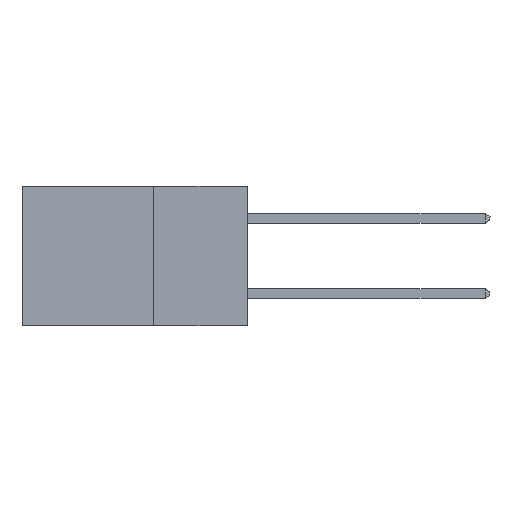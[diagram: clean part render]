
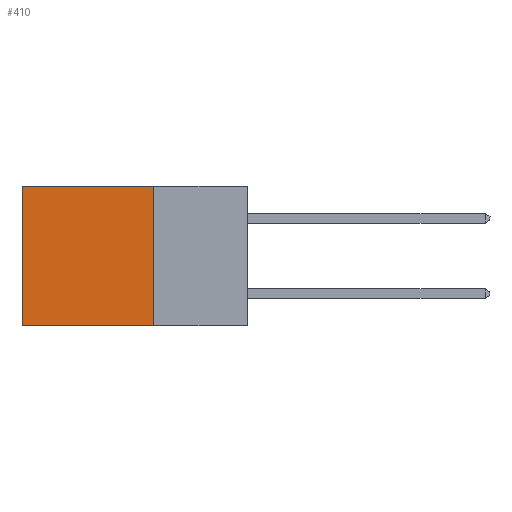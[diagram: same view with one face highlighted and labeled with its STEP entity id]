
A CAD part, left-side view. The second image highlights one B-rep face of the part: STEP entity #410.
In plain terms, the highlighted planar face has unit normal (-1, 0, 0).
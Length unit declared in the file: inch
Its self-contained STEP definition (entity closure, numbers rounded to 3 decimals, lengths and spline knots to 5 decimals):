
#233 = EDGE_CURVE ( 'NONE', #3454, #2175, #1921, .T. ) ;
#367 = DIRECTION ( 'NONE',  ( 0., 0., -1. ) ) ;
#410 = ADVANCED_FACE ( 'NONE', ( #2088 ), #538, .F. ) ;
#538 = PLANE ( 'NONE',  #8859 ) ;
#594 = VECTOR ( 'NONE', #7044, 39.37008 ) ;
#1869 = CARTESIAN_POINT ( 'NONE',  ( 0.2615, 0.6, 0. ) ) ;
#1921 = LINE ( 'NONE', #4471, #6898 ) ;
#2067 = LINE ( 'NONE', #2833, #594 ) ;
#2088 = FACE_OUTER_BOUND ( 'NONE', #9900, .T. ) ;
#2175 = VERTEX_POINT ( 'NONE', #5304 ) ;
#2203 = DIRECTION ( 'NONE',  ( 1., 0., 0. ) ) ;
#2833 = CARTESIAN_POINT ( 'NONE',  ( 0.2615, 0.6, -0.37 ) ) ;
#3124 = VECTOR ( 'NONE', #7638, 39.37008 ) ;
#3249 = EDGE_CURVE ( 'NONE', #3454, #9092, #9214, .T. ) ;
#3454 = VERTEX_POINT ( 'NONE', #5365 ) ;
#4315 = CARTESIAN_POINT ( 'NONE',  ( 0.2615, 0.25, -0.37 ) ) ;
#4471 = CARTESIAN_POINT ( 'NONE',  ( 0.2615, 0.25, -0.37 ) ) ;
#4702 = ORIENTED_EDGE ( 'NONE', *, *, #5104, .F. ) ;
#4731 = CARTESIAN_POINT ( 'NONE',  ( 0.2615, 0.6, -0.37 ) ) ;
#5104 = EDGE_CURVE ( 'NONE', #2175, #7951, #9910, .T. ) ;
#5304 = CARTESIAN_POINT ( 'NONE',  ( 0.2615, 0.25, -0.37 ) ) ;
#5365 = CARTESIAN_POINT ( 'NONE',  ( 0.2615, 0.25, 0. ) ) ;
#5917 = DIRECTION ( 'NONE',  ( 0., 1., 0. ) ) ;
#6229 = ORIENTED_EDGE ( 'NONE', *, *, #3249, .T. ) ;
#6306 = ORIENTED_EDGE ( 'NONE', *, *, #233, .F. ) ;
#6898 = VECTOR ( 'NONE', #6980, 39.37008 ) ;
#6980 = DIRECTION ( 'NONE',  ( 0., 0., -1. ) ) ;
#7044 = DIRECTION ( 'NONE',  ( 0., 0., -1. ) ) ;
#7065 = VECTOR ( 'NONE', #5917, 39.37008 ) ;
#7638 = DIRECTION ( 'NONE',  ( 0., 1., 0. ) ) ;
#7951 = VERTEX_POINT ( 'NONE', #4731 ) ;
#8197 = EDGE_CURVE ( 'NONE', #9092, #7951, #2067, .T. ) ;
#8536 = ORIENTED_EDGE ( 'NONE', *, *, #8197, .T. ) ;
#8859 = AXIS2_PLACEMENT_3D ( 'NONE', #10464, #2203, #367 ) ;
#9057 = CARTESIAN_POINT ( 'NONE',  ( 0.2615, 0.25, 0. ) ) ;
#9092 = VERTEX_POINT ( 'NONE', #1869 ) ;
#9214 = LINE ( 'NONE', #9057, #7065 ) ;
#9900 = EDGE_LOOP ( 'NONE', ( #8536, #4702, #6306, #6229 ) ) ;
#9910 = LINE ( 'NONE', #4315, #3124 ) ;
#10464 = CARTESIAN_POINT ( 'NONE',  ( 0.2615, 0.25, -0.37 ) ) ;
